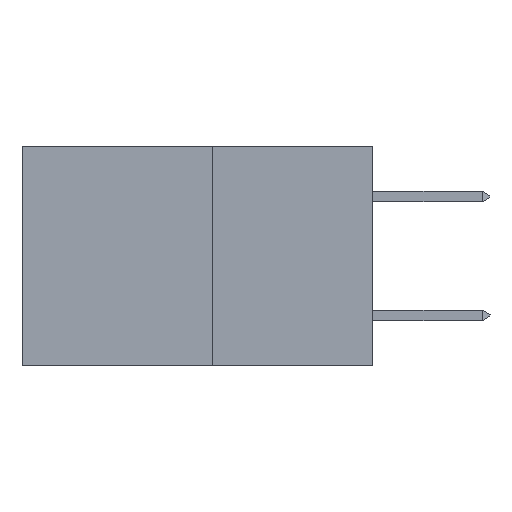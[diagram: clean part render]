
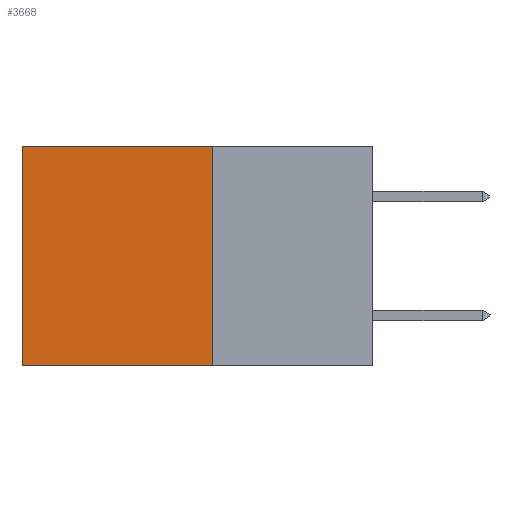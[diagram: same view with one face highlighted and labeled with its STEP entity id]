
A CAD part, left-side view. The second image highlights one B-rep face of the part: STEP entity #3668.
In plain terms, the highlighted planar face has unit normal (-1, 0, 0).
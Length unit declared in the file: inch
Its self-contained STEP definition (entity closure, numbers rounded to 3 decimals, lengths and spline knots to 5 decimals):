
#319 = VECTOR ( 'NONE', #15629, 39.37008 ) ;
#350 = VECTOR ( 'NONE', #7539, 39.37008 ) ;
#721 = AXIS2_PLACEMENT_3D ( 'NONE', #15143, #10249, #20341 ) ;
#1458 = ORIENTED_EDGE ( 'NONE', *, *, #11444, .F. ) ;
#1556 = VERTEX_POINT ( 'NONE', #4714 ) ;
#1616 = VECTOR ( 'NONE', #14151, 39.37008 ) ;
#2415 = CARTESIAN_POINT ( 'NONE',  ( 0.277, 0.27, -0.37 ) ) ;
#3668 = ADVANCED_FACE ( 'NONE', ( #17956 ), #12789, .F. ) ;
#4344 = LINE ( 'NONE', #17881, #4871 ) ;
#4429 = LINE ( 'NONE', #6702, #319 ) ;
#4714 = CARTESIAN_POINT ( 'NONE',  ( 0.277, 0.59, -0.37 ) ) ;
#4742 = CARTESIAN_POINT ( 'NONE',  ( 0.277, 0.59, 0. ) ) ;
#4871 = VECTOR ( 'NONE', #18657, 39.37008 ) ;
#5336 = VERTEX_POINT ( 'NONE', #4742 ) ;
#6702 = CARTESIAN_POINT ( 'NONE',  ( 0.277, 0.27, 0. ) ) ;
#7191 = ORIENTED_EDGE ( 'NONE', *, *, #7902, .F. ) ;
#7539 = DIRECTION ( 'NONE',  ( 0., 1., 0. ) ) ;
#7553 = CARTESIAN_POINT ( 'NONE',  ( 0.277, 0.27, -0.37 ) ) ;
#7768 = EDGE_CURVE ( 'NONE', #5336, #1556, #4344, .T. ) ;
#7902 = EDGE_CURVE ( 'NONE', #14653, #14611, #15166, .T. ) ;
#10249 = DIRECTION ( 'NONE',  ( 1., 0., 0. ) ) ;
#11444 = EDGE_CURVE ( 'NONE', #14611, #1556, #18430, .T. ) ;
#12789 = PLANE ( 'NONE',  #721 ) ;
#12849 = EDGE_LOOP ( 'NONE', ( #15698, #1458, #7191, #18630 ) ) ;
#13554 = CARTESIAN_POINT ( 'NONE',  ( 0.277, 0.27, -0.37 ) ) ;
#13789 = EDGE_CURVE ( 'NONE', #14653, #5336, #4429, .T. ) ;
#14151 = DIRECTION ( 'NONE',  ( 0., 0., -1. ) ) ;
#14611 = VERTEX_POINT ( 'NONE', #7553 ) ;
#14653 = VERTEX_POINT ( 'NONE', #19382 ) ;
#15143 = CARTESIAN_POINT ( 'NONE',  ( 0.277, 0.27, -0.37 ) ) ;
#15166 = LINE ( 'NONE', #13554, #1616 ) ;
#15629 = DIRECTION ( 'NONE',  ( 0., 1., 0. ) ) ;
#15698 = ORIENTED_EDGE ( 'NONE', *, *, #7768, .T. ) ;
#17881 = CARTESIAN_POINT ( 'NONE',  ( 0.277, 0.59, -0.37 ) ) ;
#17956 = FACE_OUTER_BOUND ( 'NONE', #12849, .T. ) ;
#18430 = LINE ( 'NONE', #2415, #350 ) ;
#18630 = ORIENTED_EDGE ( 'NONE', *, *, #13789, .T. ) ;
#18657 = DIRECTION ( 'NONE',  ( 0., 0., -1. ) ) ;
#19382 = CARTESIAN_POINT ( 'NONE',  ( 0.277, 0.27, 0. ) ) ;
#20341 = DIRECTION ( 'NONE',  ( 0., 0., -1. ) ) ;
